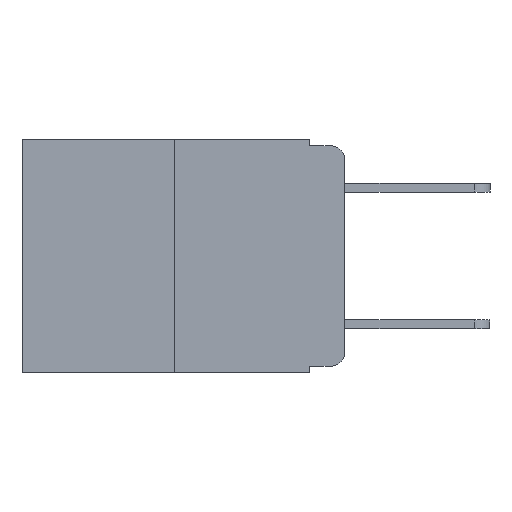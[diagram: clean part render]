
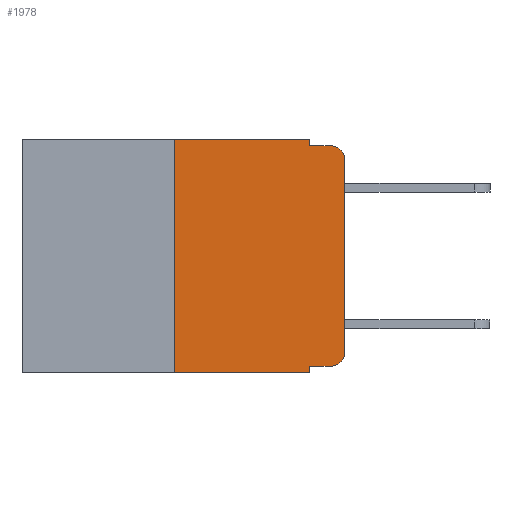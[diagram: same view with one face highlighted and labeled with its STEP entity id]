
A CAD part, left-side view. The second image highlights one B-rep face of the part: STEP entity #1978.
In plain terms, the highlighted planar face has unit normal (-1, 0, 0).
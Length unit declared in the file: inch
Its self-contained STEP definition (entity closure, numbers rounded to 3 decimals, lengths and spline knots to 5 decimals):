
#192 = VECTOR ( 'NONE', #7324, 39.37008 ) ;
#357 = VECTOR ( 'NONE', #18570, 39.37008 ) ;
#642 = DIRECTION ( 'NONE',  ( 0., 0., -1. ) ) ;
#666 = VERTEX_POINT ( 'NONE', #14614 ) ;
#763 = VECTOR ( 'NONE', #19939, 39.37008 ) ;
#1817 = CARTESIAN_POINT ( 'NONE',  ( 0., 0.051, -0.333 ) ) ;
#1915 = LINE ( 'NONE', #16846, #14746 ) ;
#1978 = ADVANCED_FACE ( 'NONE', ( #14766 ), #14204, .F. ) ;
#2046 = CARTESIAN_POINT ( 'NONE',  ( 0., 0.051, -0.343 ) ) ;
#2135 = ORIENTED_EDGE ( 'NONE', *, *, #16445, .T. ) ;
#2307 = CARTESIAN_POINT ( 'NONE',  ( 0., 0.473, -0.343 ) ) ;
#2386 = CARTESIAN_POINT ( 'NONE',  ( 0., 0.051, 0. ) ) ;
#2547 = LINE ( 'NONE', #15728, #19226 ) ;
#3166 = EDGE_CURVE ( 'NONE', #12288, #13781, #1915, .T. ) ;
#4062 = CARTESIAN_POINT ( 'NONE',  ( 0., 0.051, 0. ) ) ;
#4146 = CARTESIAN_POINT ( 'NONE',  ( 0., 0.25, -0.343 ) ) ;
#4278 = ORIENTED_EDGE ( 'NONE', *, *, #10611, .T. ) ;
#4349 = VERTEX_POINT ( 'NONE', #16103 ) ;
#4427 = LINE ( 'NONE', #8333, #12257 ) ;
#4509 = VERTEX_POINT ( 'NONE', #5186 ) ;
#4766 = VERTEX_POINT ( 'NONE', #4146 ) ;
#4867 = LINE ( 'NONE', #18499, #357 ) ;
#5186 = CARTESIAN_POINT ( 'NONE',  ( 0., 0., -0.313 ) ) ;
#5408 = CIRCLE ( 'NONE', #17325, 0.02 ) ;
#5431 = VERTEX_POINT ( 'NONE', #5953 ) ;
#5578 = EDGE_CURVE ( 'NONE', #666, #4509, #18070, .T. ) ;
#5828 = CARTESIAN_POINT ( 'NONE',  ( 0., 0.02, -0.03 ) ) ;
#5953 = CARTESIAN_POINT ( 'NONE',  ( 0., 0.25, 0. ) ) ;
#6268 = DIRECTION ( 'NONE',  ( 0., -1., 0. ) ) ;
#6746 = VECTOR ( 'NONE', #15773, 39.37008 ) ;
#6843 = LINE ( 'NONE', #13305, #763 ) ;
#7039 = LINE ( 'NONE', #4062, #11985 ) ;
#7049 = CARTESIAN_POINT ( 'NONE',  ( 0., 0.02, -0.01 ) ) ;
#7107 = EDGE_LOOP ( 'NONE', ( #2135, #4278, #11866, #8235, #17859, #16559, #9042, #11147, #13737, #11929 ) ) ;
#7324 = DIRECTION ( 'NONE',  ( 0., -1., 0. ) ) ;
#7505 = DIRECTION ( 'NONE',  ( 0., 0., -1. ) ) ;
#8120 = LINE ( 'NONE', #2307, #192 ) ;
#8235 = ORIENTED_EDGE ( 'NONE', *, *, #15730, .F. ) ;
#8333 = CARTESIAN_POINT ( 'NONE',  ( 0., 0.051, -0.333 ) ) ;
#8623 = EDGE_CURVE ( 'NONE', #4766, #9141, #8120, .T. ) ;
#9042 = ORIENTED_EDGE ( 'NONE', *, *, #8623, .T. ) ;
#9141 = VERTEX_POINT ( 'NONE', #2046 ) ;
#9612 = VERTEX_POINT ( 'NONE', #1817 ) ;
#9747 = DIRECTION ( 'NONE',  ( -1., 0., 0. ) ) ;
#10611 = EDGE_CURVE ( 'NONE', #4349, #13781, #5408, .T. ) ;
#11147 = ORIENTED_EDGE ( 'NONE', *, *, #15114, .F. ) ;
#11301 = DIRECTION ( 'NONE',  ( 1., 0., 0. ) ) ;
#11706 = LINE ( 'NONE', #2386, #6746 ) ;
#11866 = ORIENTED_EDGE ( 'NONE', *, *, #3166, .F. ) ;
#11881 = CARTESIAN_POINT ( 'NONE',  ( 0., 0.051, -0.01 ) ) ;
#11929 = ORIENTED_EDGE ( 'NONE', *, *, #5578, .T. ) ;
#11985 = VECTOR ( 'NONE', #642, 39.37008 ) ;
#12118 = AXIS2_PLACEMENT_3D ( 'NONE', #19643, #9747, #21288 ) ;
#12257 = VECTOR ( 'NONE', #19899, 39.37008 ) ;
#12288 = VERTEX_POINT ( 'NONE', #11881 ) ;
#12680 = DIRECTION ( 'NONE',  ( 0., 0., -1. ) ) ;
#13305 = CARTESIAN_POINT ( 'NONE',  ( 0., 0.473, 0. ) ) ;
#13591 = CARTESIAN_POINT ( 'NONE',  ( 0., 0.051, 0. ) ) ;
#13653 = EDGE_CURVE ( 'NONE', #5431, #13756, #6843, .T. ) ;
#13737 = ORIENTED_EDGE ( 'NONE', *, *, #14820, .T. ) ;
#13756 = VERTEX_POINT ( 'NONE', #13591 ) ;
#13781 = VERTEX_POINT ( 'NONE', #7049 ) ;
#14204 = PLANE ( 'NONE',  #15487 ) ;
#14614 = CARTESIAN_POINT ( 'NONE',  ( 0., 0.02, -0.333 ) ) ;
#14746 = VECTOR ( 'NONE', #6268, 39.37008 ) ;
#14766 = FACE_OUTER_BOUND ( 'NONE', #7107, .T. ) ;
#14769 = CARTESIAN_POINT ( 'NONE',  ( 0., 0.473, 0. ) ) ;
#14820 = EDGE_CURVE ( 'NONE', #9612, #666, #4427, .T. ) ;
#15114 = EDGE_CURVE ( 'NONE', #9612, #9141, #7039, .T. ) ;
#15145 = EDGE_CURVE ( 'NONE', #4766, #5431, #2547, .T. ) ;
#15487 = AXIS2_PLACEMENT_3D ( 'NONE', #14769, #11301, #12680 ) ;
#15728 = CARTESIAN_POINT ( 'NONE',  ( 0., 0.25, 0. ) ) ;
#15730 = EDGE_CURVE ( 'NONE', #13756, #12288, #11706, .T. ) ;
#15773 = DIRECTION ( 'NONE',  ( 0., 0., -1. ) ) ;
#16103 = CARTESIAN_POINT ( 'NONE',  ( 0., 0., -0.03 ) ) ;
#16445 = EDGE_CURVE ( 'NONE', #4509, #4349, #4867, .T. ) ;
#16559 = ORIENTED_EDGE ( 'NONE', *, *, #15145, .F. ) ;
#16846 = CARTESIAN_POINT ( 'NONE',  ( 0., 0.051, -0.01 ) ) ;
#17325 = AXIS2_PLACEMENT_3D ( 'NONE', #5828, #17454, #7505 ) ;
#17454 = DIRECTION ( 'NONE',  ( -1., 0., 0. ) ) ;
#17859 = ORIENTED_EDGE ( 'NONE', *, *, #13653, .F. ) ;
#18070 = CIRCLE ( 'NONE', #12118, 0.02 ) ;
#18499 = CARTESIAN_POINT ( 'NONE',  ( 0., 0., 0. ) ) ;
#18570 = DIRECTION ( 'NONE',  ( 0., 0., 1. ) ) ;
#19226 = VECTOR ( 'NONE', #20662, 39.37008 ) ;
#19643 = CARTESIAN_POINT ( 'NONE',  ( 0., 0.02, -0.313 ) ) ;
#19899 = DIRECTION ( 'NONE',  ( 0., -1., 0. ) ) ;
#19939 = DIRECTION ( 'NONE',  ( 0., -1., 0. ) ) ;
#20662 = DIRECTION ( 'NONE',  ( 0., 0., 1. ) ) ;
#21288 = DIRECTION ( 'NONE',  ( 0., 0., -1. ) ) ;
